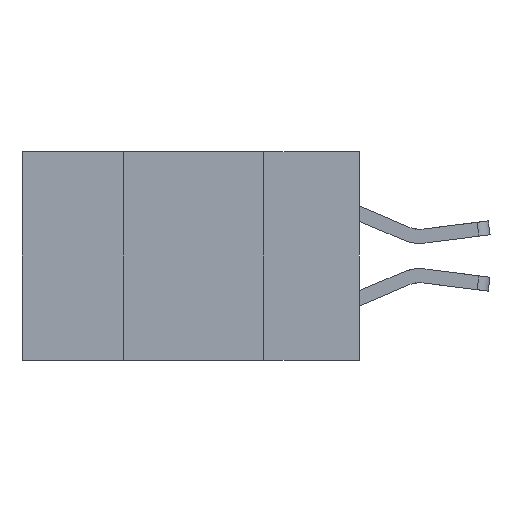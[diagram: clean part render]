
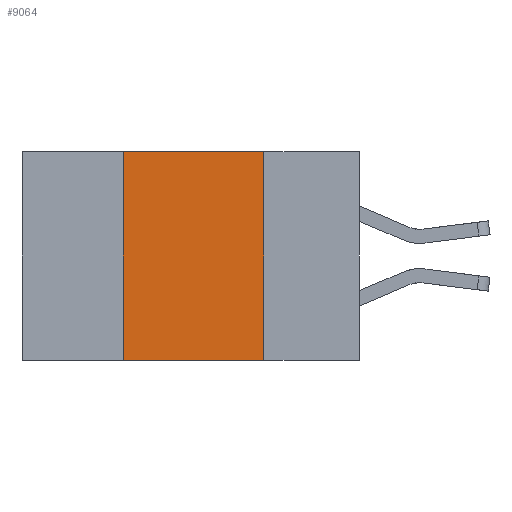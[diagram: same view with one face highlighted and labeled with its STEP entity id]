
A CAD part, left-side view. The second image highlights one B-rep face of the part: STEP entity #9064.
In plain terms, the highlighted planar face has unit normal (-1, 0, 0).
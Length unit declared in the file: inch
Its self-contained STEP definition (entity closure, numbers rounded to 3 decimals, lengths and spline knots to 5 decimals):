
#9 = VECTOR ( 'NONE', #4360, 39.37008 ) ;
#383 = VERTEX_POINT ( 'NONE', #11934 ) ;
#436 = LINE ( 'NONE', #12345, #9 ) ;
#890 = VECTOR ( 'NONE', #6592, 39.37008 ) ;
#907 = CARTESIAN_POINT ( 'NONE',  ( 0., 0.17, -0.37 ) ) ;
#1317 = CARTESIAN_POINT ( 'NONE',  ( 0., 0.6, 0. ) ) ;
#2621 = VERTEX_POINT ( 'NONE', #4056 ) ;
#3283 = EDGE_CURVE ( 'NONE', #2621, #383, #11303, .T. ) ;
#3402 = AXIS2_PLACEMENT_3D ( 'NONE', #8238, #11279, #8304 ) ;
#4056 = CARTESIAN_POINT ( 'NONE',  ( 0., 0.42, 0. ) ) ;
#4358 = CARTESIAN_POINT ( 'NONE',  ( 0., 0.42, 0. ) ) ;
#4360 = DIRECTION ( 'NONE',  ( 0., -1., 0. ) ) ;
#4424 = VERTEX_POINT ( 'NONE', #907 ) ;
#5137 = PLANE ( 'NONE',  #3402 ) ;
#5505 = VERTEX_POINT ( 'NONE', #9320 ) ;
#5907 = ORIENTED_EDGE ( 'NONE', *, *, #3283, .F. ) ;
#5915 = EDGE_CURVE ( 'NONE', #5505, #2621, #12528, .T. ) ;
#6592 = DIRECTION ( 'NONE',  ( 0., 0., -1. ) ) ;
#7225 = EDGE_CURVE ( 'NONE', #5505, #4424, #436, .T. ) ;
#7728 = VECTOR ( 'NONE', #12656, 39.37008 ) ;
#8238 = CARTESIAN_POINT ( 'NONE',  ( 0., 0.6, 0. ) ) ;
#8304 = DIRECTION ( 'NONE',  ( 0., 0., -1. ) ) ;
#9064 = ADVANCED_FACE ( 'NONE', ( #10886 ), #5137, .F. ) ;
#9320 = CARTESIAN_POINT ( 'NONE',  ( 0., 0.42, -0.37 ) ) ;
#9576 = LINE ( 'NONE', #12600, #890 ) ;
#9608 = ORIENTED_EDGE ( 'NONE', *, *, #7225, .T. ) ;
#9875 = EDGE_LOOP ( 'NONE', ( #12451, #5907, #10821, #9608 ) ) ;
#10821 = ORIENTED_EDGE ( 'NONE', *, *, #5915, .F. ) ;
#10886 = FACE_OUTER_BOUND ( 'NONE', #9875, .T. ) ;
#11279 = DIRECTION ( 'NONE',  ( 1., 0., 0. ) ) ;
#11303 = LINE ( 'NONE', #1317, #7728 ) ;
#11413 = DIRECTION ( 'NONE',  ( 0., 0., 1. ) ) ;
#11934 = CARTESIAN_POINT ( 'NONE',  ( 0., 0.17, 0. ) ) ;
#12345 = CARTESIAN_POINT ( 'NONE',  ( 0., 0.6, -0.37 ) ) ;
#12451 = ORIENTED_EDGE ( 'NONE', *, *, #12794, .F. ) ;
#12528 = LINE ( 'NONE', #4358, #12919 ) ;
#12600 = CARTESIAN_POINT ( 'NONE',  ( 0., 0.17, 0. ) ) ;
#12656 = DIRECTION ( 'NONE',  ( 0., -1., 0. ) ) ;
#12794 = EDGE_CURVE ( 'NONE', #383, #4424, #9576, .T. ) ;
#12919 = VECTOR ( 'NONE', #11413, 39.37008 ) ;
